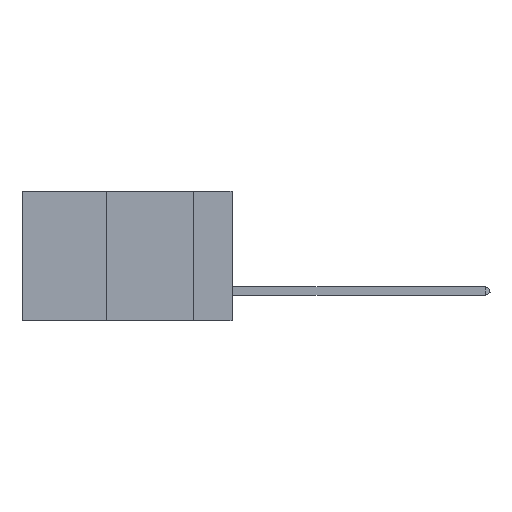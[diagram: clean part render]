
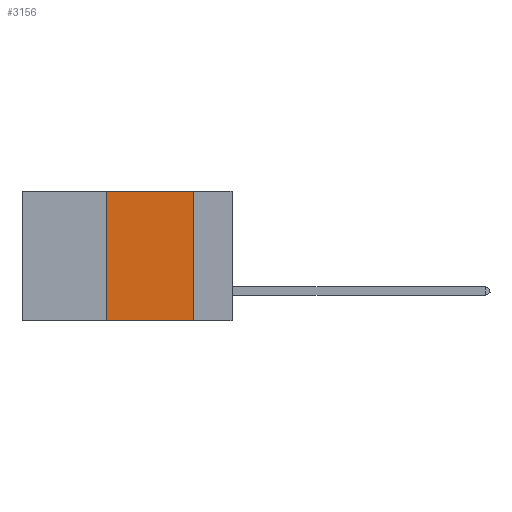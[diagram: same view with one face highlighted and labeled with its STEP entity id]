
A CAD part, left-side view. The second image highlights one B-rep face of the part: STEP entity #3156.
In plain terms, the highlighted planar face has unit normal (-1, 0, 0).
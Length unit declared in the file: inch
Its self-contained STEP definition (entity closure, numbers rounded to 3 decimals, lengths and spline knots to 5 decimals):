
#288 = EDGE_CURVE ( 'NONE', #13331, #17836, #3279, .T. ) ;
#449 = ORIENTED_EDGE ( 'NONE', *, *, #2815, .T. ) ;
#1304 = DIRECTION ( 'NONE',  ( 0., -1., 0. ) ) ;
#2772 = CARTESIAN_POINT ( 'NONE',  ( 0., 0.36, 0. ) ) ;
#2815 = EDGE_CURVE ( 'NONE', #3912, #17836, #3214, .T. ) ;
#3156 = ADVANCED_FACE ( 'NONE', ( #18437 ), #5344, .F. ) ;
#3214 = LINE ( 'NONE', #13272, #8280 ) ;
#3223 = EDGE_CURVE ( 'NONE', #18121, #13331, #12670, .T. ) ;
#3279 = LINE ( 'NONE', #17765, #13219 ) ;
#3912 = VERTEX_POINT ( 'NONE', #16735 ) ;
#4202 = DIRECTION ( 'NONE',  ( 1., 0., 0. ) ) ;
#4513 = DIRECTION ( 'NONE',  ( 0., -1., 0. ) ) ;
#4528 = VECTOR ( 'NONE', #1304, 39.37008 ) ;
#5344 = PLANE ( 'NONE',  #15342 ) ;
#5667 = EDGE_CURVE ( 'NONE', #3912, #18121, #12640, .T. ) ;
#8280 = VECTOR ( 'NONE', #4513, 39.37008 ) ;
#8299 = CARTESIAN_POINT ( 'NONE',  ( 0., 0.11, 0. ) ) ;
#8555 = ORIENTED_EDGE ( 'NONE', *, *, #5667, .F. ) ;
#10740 = EDGE_LOOP ( 'NONE', ( #11380, #14916, #8555, #449 ) ) ;
#11082 = DIRECTION ( 'NONE',  ( 0., 0., -1. ) ) ;
#11234 = DIRECTION ( 'NONE',  ( 0., 0., 1. ) ) ;
#11380 = ORIENTED_EDGE ( 'NONE', *, *, #288, .F. ) ;
#11441 = VECTOR ( 'NONE', #11234, 39.37008 ) ;
#12640 = LINE ( 'NONE', #2772, #11441 ) ;
#12670 = LINE ( 'NONE', #17291, #4528 ) ;
#13219 = VECTOR ( 'NONE', #14578, 39.37008 ) ;
#13258 = CARTESIAN_POINT ( 'NONE',  ( 0., 0.36, 0. ) ) ;
#13272 = CARTESIAN_POINT ( 'NONE',  ( 0., 0.6, -0.37 ) ) ;
#13331 = VERTEX_POINT ( 'NONE', #8299 ) ;
#13654 = CARTESIAN_POINT ( 'NONE',  ( 0., 0.11, -0.37 ) ) ;
#14091 = CARTESIAN_POINT ( 'NONE',  ( 0., 0.6, 0. ) ) ;
#14578 = DIRECTION ( 'NONE',  ( 0., 0., -1. ) ) ;
#14916 = ORIENTED_EDGE ( 'NONE', *, *, #3223, .F. ) ;
#15342 = AXIS2_PLACEMENT_3D ( 'NONE', #14091, #4202, #11082 ) ;
#16735 = CARTESIAN_POINT ( 'NONE',  ( 0., 0.36, -0.37 ) ) ;
#17291 = CARTESIAN_POINT ( 'NONE',  ( 0., 0.6, 0. ) ) ;
#17765 = CARTESIAN_POINT ( 'NONE',  ( 0., 0.11, 0. ) ) ;
#17836 = VERTEX_POINT ( 'NONE', #13654 ) ;
#18121 = VERTEX_POINT ( 'NONE', #13258 ) ;
#18437 = FACE_OUTER_BOUND ( 'NONE', #10740, .T. ) ;
